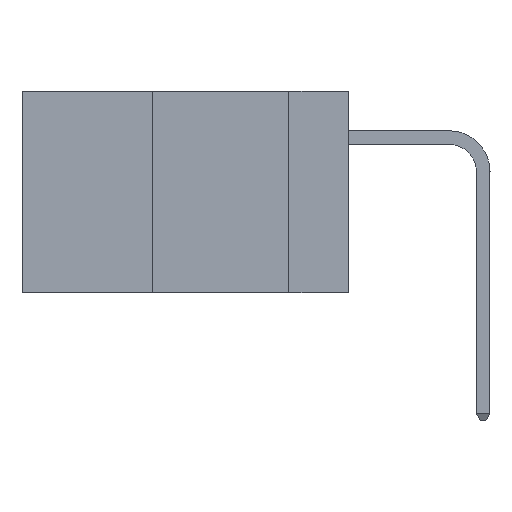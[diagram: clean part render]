
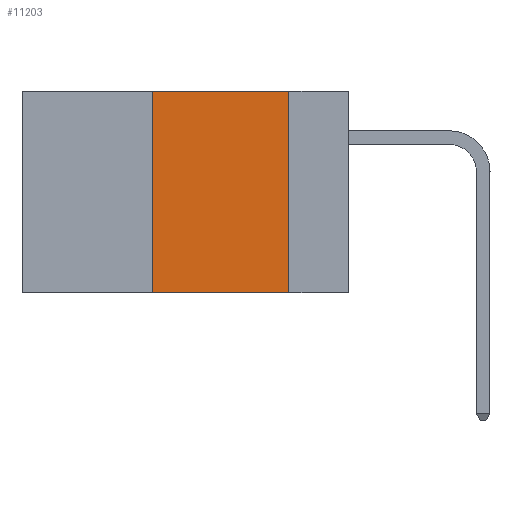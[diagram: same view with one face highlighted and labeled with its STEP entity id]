
A CAD part, left-side view. The second image highlights one B-rep face of the part: STEP entity #11203.
In plain terms, the highlighted planar face has unit normal (-1, 0, 0).
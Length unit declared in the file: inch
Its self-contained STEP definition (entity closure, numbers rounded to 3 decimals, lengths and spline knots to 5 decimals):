
#55 = ORIENTED_EDGE ( 'NONE', *, *, #983, .F. ) ;
#262 = VECTOR ( 'NONE', #7400, 39.37008 ) ;
#370 = EDGE_CURVE ( 'NONE', #5611, #7833, #8680, .T. ) ;
#498 = LINE ( 'NONE', #3951, #262 ) ;
#543 = ORIENTED_EDGE ( 'NONE', *, *, #370, .F. ) ;
#565 = VERTEX_POINT ( 'NONE', #5327 ) ;
#831 = VECTOR ( 'NONE', #6821, 39.37008 ) ;
#983 = EDGE_CURVE ( 'NONE', #7455, #5611, #8718, .T. ) ;
#1018 = VECTOR ( 'NONE', #9767, 39.37008 ) ;
#1126 = VECTOR ( 'NONE', #1723, 39.37008 ) ;
#1695 = EDGE_CURVE ( 'NONE', #7455, #565, #2484, .T. ) ;
#1723 = DIRECTION ( 'NONE',  ( 0., -1., 0. ) ) ;
#2484 = LINE ( 'NONE', #3438, #831 ) ;
#2986 = CARTESIAN_POINT ( 'NONE',  ( 0., 0.36, -0.37 ) ) ;
#3012 = CARTESIAN_POINT ( 'NONE',  ( 0., 0.6, 0. ) ) ;
#3438 = CARTESIAN_POINT ( 'NONE',  ( 0., 0.6, -0.37 ) ) ;
#3951 = CARTESIAN_POINT ( 'NONE',  ( 0., 0.11, 0. ) ) ;
#4785 = ORIENTED_EDGE ( 'NONE', *, *, #7360, .F. ) ;
#5327 = CARTESIAN_POINT ( 'NONE',  ( 0., 0.11, -0.37 ) ) ;
#5478 = DIRECTION ( 'NONE',  ( 1., 0., 0. ) ) ;
#5611 = VERTEX_POINT ( 'NONE', #6994 ) ;
#6821 = DIRECTION ( 'NONE',  ( 0., -1., 0. ) ) ;
#6994 = CARTESIAN_POINT ( 'NONE',  ( 0., 0.36, 0. ) ) ;
#7021 = CARTESIAN_POINT ( 'NONE',  ( 0., 0.36, 0. ) ) ;
#7187 = PLANE ( 'NONE',  #10464 ) ;
#7332 = CARTESIAN_POINT ( 'NONE',  ( 0., 0.11, 0. ) ) ;
#7360 = EDGE_CURVE ( 'NONE', #7833, #565, #498, .T. ) ;
#7400 = DIRECTION ( 'NONE',  ( 0., 0., -1. ) ) ;
#7455 = VERTEX_POINT ( 'NONE', #2986 ) ;
#7833 = VERTEX_POINT ( 'NONE', #7332 ) ;
#8041 = FACE_OUTER_BOUND ( 'NONE', #10018, .T. ) ;
#8680 = LINE ( 'NONE', #10353, #1126 ) ;
#8684 = ORIENTED_EDGE ( 'NONE', *, *, #1695, .T. ) ;
#8718 = LINE ( 'NONE', #7021, #1018 ) ;
#9767 = DIRECTION ( 'NONE',  ( 0., 0., 1. ) ) ;
#10018 = EDGE_LOOP ( 'NONE', ( #4785, #543, #55, #8684 ) ) ;
#10353 = CARTESIAN_POINT ( 'NONE',  ( 0., 0.6, 0. ) ) ;
#10464 = AXIS2_PLACEMENT_3D ( 'NONE', #3012, #5478, #10742 ) ;
#10742 = DIRECTION ( 'NONE',  ( 0., 0., -1. ) ) ;
#11203 = ADVANCED_FACE ( 'NONE', ( #8041 ), #7187, .F. ) ;
